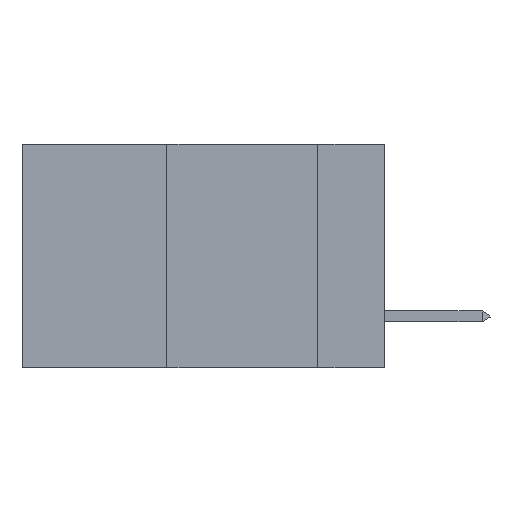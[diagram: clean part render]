
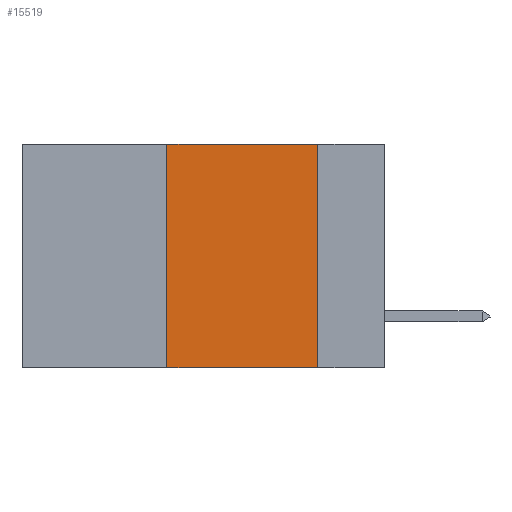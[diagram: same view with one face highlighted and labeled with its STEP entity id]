
A CAD part, left-side view. The second image highlights one B-rep face of the part: STEP entity #15519.
In plain terms, the highlighted planar face has unit normal (-1, 0, 0).
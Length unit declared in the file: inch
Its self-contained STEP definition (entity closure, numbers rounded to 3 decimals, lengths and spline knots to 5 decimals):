
#496 = CARTESIAN_POINT ( 'NONE',  ( 0., 0.36, 0. ) ) ;
#1223 = CARTESIAN_POINT ( 'NONE',  ( 0., 0.6, 0. ) ) ;
#2009 = EDGE_CURVE ( 'NONE', #5465, #17626, #14966, .T. ) ;
#2506 = EDGE_CURVE ( 'NONE', #8447, #17626, #10302, .T. ) ;
#2797 = DIRECTION ( 'NONE',  ( 0., -1., 0. ) ) ;
#3638 = DIRECTION ( 'NONE',  ( 0., 0., 1. ) ) ;
#3788 = LINE ( 'NONE', #1223, #15296 ) ;
#5324 = CARTESIAN_POINT ( 'NONE',  ( 0., 0.36, -0.37 ) ) ;
#5447 = EDGE_CURVE ( 'NONE', #6667, #5465, #3788, .T. ) ;
#5465 = VERTEX_POINT ( 'NONE', #14990 ) ;
#6050 = ORIENTED_EDGE ( 'NONE', *, *, #5447, .F. ) ;
#6100 = VECTOR ( 'NONE', #14087, 39.37008 ) ;
#6667 = VERTEX_POINT ( 'NONE', #496 ) ;
#7218 = CARTESIAN_POINT ( 'NONE',  ( 0., 0.11, -0.37 ) ) ;
#8217 = CARTESIAN_POINT ( 'NONE',  ( 0., 0.36, 0. ) ) ;
#8233 = VECTOR ( 'NONE', #3638, 39.37008 ) ;
#8447 = VERTEX_POINT ( 'NONE', #5324 ) ;
#8697 = CARTESIAN_POINT ( 'NONE',  ( 0., 0.6, -0.37 ) ) ;
#9031 = DIRECTION ( 'NONE',  ( 0., 0., -1. ) ) ;
#9892 = PLANE ( 'NONE',  #18695 ) ;
#10302 = LINE ( 'NONE', #8697, #12850 ) ;
#11666 = CARTESIAN_POINT ( 'NONE',  ( 0., 0.11, 0. ) ) ;
#12240 = ORIENTED_EDGE ( 'NONE', *, *, #19121, .F. ) ;
#12260 = ORIENTED_EDGE ( 'NONE', *, *, #2506, .T. ) ;
#12850 = VECTOR ( 'NONE', #19198, 39.37008 ) ;
#13517 = CARTESIAN_POINT ( 'NONE',  ( 0., 0.6, 0. ) ) ;
#13694 = EDGE_LOOP ( 'NONE', ( #14342, #6050, #12240, #12260 ) ) ;
#14087 = DIRECTION ( 'NONE',  ( 0., 0., -1. ) ) ;
#14342 = ORIENTED_EDGE ( 'NONE', *, *, #2009, .F. ) ;
#14966 = LINE ( 'NONE', #11666, #6100 ) ;
#14990 = CARTESIAN_POINT ( 'NONE',  ( 0., 0.11, 0. ) ) ;
#15221 = DIRECTION ( 'NONE',  ( 1., 0., 0. ) ) ;
#15296 = VECTOR ( 'NONE', #2797, 39.37008 ) ;
#15519 = ADVANCED_FACE ( 'NONE', ( #16528 ), #9892, .F. ) ;
#16528 = FACE_OUTER_BOUND ( 'NONE', #13694, .T. ) ;
#16865 = LINE ( 'NONE', #8217, #8233 ) ;
#17626 = VERTEX_POINT ( 'NONE', #7218 ) ;
#18695 = AXIS2_PLACEMENT_3D ( 'NONE', #13517, #15221, #9031 ) ;
#19121 = EDGE_CURVE ( 'NONE', #8447, #6667, #16865, .T. ) ;
#19198 = DIRECTION ( 'NONE',  ( 0., -1., 0. ) ) ;
